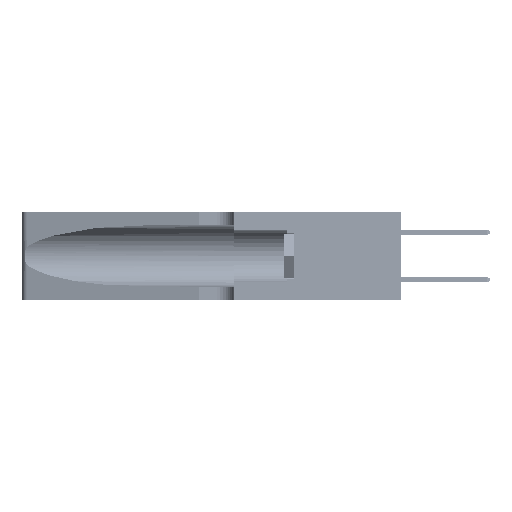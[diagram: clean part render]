
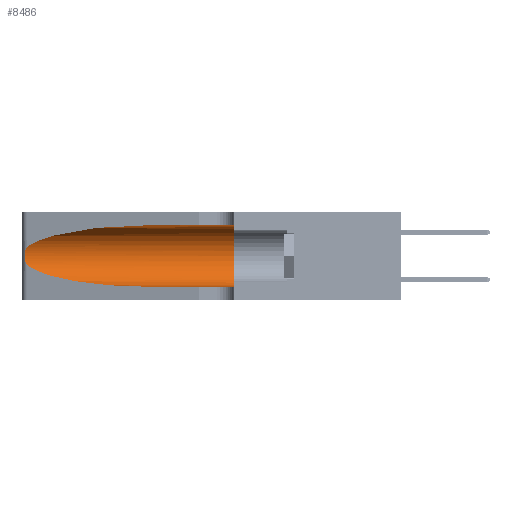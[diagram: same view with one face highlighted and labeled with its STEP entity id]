
A CAD part, left-side view. The second image highlights one B-rep face of the part: STEP entity #8486.
In plain terms, the highlighted cylindrical face has radius 3.308 mm (diameter 6.617 mm), a partial arc.
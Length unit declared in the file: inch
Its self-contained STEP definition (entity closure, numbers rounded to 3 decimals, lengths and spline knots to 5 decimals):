
#449 = CARTESIAN_POINT ( 'NONE',  ( 0.25487, 1.22718, 0.22369 ) ) ;
#981 = VERTEX_POINT ( 'NONE', #46132 ) ;
#1386 = CARTESIAN_POINT ( 'NONE',  ( 0.1305, 0.72297, 0.05475 ) ) ;
#2891 = CARTESIAN_POINT ( 'NONE',  ( 0.26017, 1.23833, 0.17102 ) ) ;
#5799 = CARTESIAN_POINT ( 'NONE',  ( 0.1305, 0.72297, 0.31525 ) ) ;
#6157 = VERTEX_POINT ( 'NONE', #449 ) ;
#6566 = CARTESIAN_POINT ( 'NONE',  ( 0.1305, 1.61858, 0.05475 ) ) ;
#7094 = CARTESIAN_POINT ( 'NONE',  ( 0.25789, 1.23486, 0.15765 ) ) ;
#7376 = CARTESIAN_POINT ( 'NONE',  ( 0.1305, 0.35, 0.185 ) ) ;
#8252 = CARTESIAN_POINT ( 'NONE',  ( 0.1305, 1.61858, 0.31525 ) ) ;
#8486 = ADVANCED_FACE ( 'NONE', ( #23718 ), #43010, .F. ) ;
#9525 = EDGE_CURVE ( 'NONE', #6157, #41247, #24812, .T. ) ;
#10135 = LINE ( 'NONE', #6566, #51354 ) ;
#10443 = ORIENTED_EDGE ( 'NONE', *, *, #43937, .F. ) ;
#10469 = CARTESIAN_POINT ( 'NONE',  ( 0.25487, 1.22718, 0.14631 ) ) ;
#11297 = CARTESIAN_POINT ( 'NONE',  ( 0.25555, 1.22993, 0.14849 ) ) ;
#11585 = DIRECTION ( 'NONE',  ( 0., 0., 1. ) ) ;
#13323 = EDGE_CURVE ( 'NONE', #981, #30240, #10135, .T. ) ;
#14059 = CARTESIAN_POINT ( 'NONE',  ( 0.1305, 0.72297, 0.31525 ) ) ;
#15087 = CARTESIAN_POINT ( 'NONE',  ( 0.25555, 1.22994, 0.2215 ) ) ;
#17076 = EDGE_CURVE ( 'NONE', #32640, #30240, #30531, .T. ) ;
#17966 = CARTESIAN_POINT ( 'NONE',  ( 0.25487, 1.22718, 0.14631 ) ) ;
#19010 = CARTESIAN_POINT ( 'NONE',  ( 0.1305, 1.61858, 0.185 ) ) ;
#19430 = CARTESIAN_POINT ( 'NONE',  ( 0.25787, 1.23484, 0.2124 ) ) ;
#22387 = CARTESIAN_POINT ( 'NONE',  ( 0.25487, 1.22718, 0.22369 ) ) ;
#23558 = CARTESIAN_POINT ( 'NONE',  ( 0.26018, 1.23835, 0.19895 ) ) ;
#23718 = FACE_OUTER_BOUND ( 'NONE', #50709, .T. ) ;
#24812 = B_SPLINE_CURVE_WITH_KNOTS ( 'NONE', 3,
 ( #35809, #15087, #44046, #19430, #48193, #23558, #52320, #27721, #2891, #31877, #7094, #35980, #11297, #40113 ),
 .UNSPECIFIED., .F., .F.,
 ( 4, 2, 2, 2, 2, 2, 4 ),
 ( 0., 0.00027, 0.00053, 0.00107, 0.0016, 0.00187, 0.00214 ),
 .UNSPECIFIED. ) ;
#25720 = ORIENTED_EDGE ( 'NONE', *, *, #41155, .T. ) ;
#26239 = CARTESIAN_POINT ( 'NONE',  ( 0.18966, 0.96281, 0.05475 ) ) ;
#27721 = CARTESIAN_POINT ( 'NONE',  ( 0.26075, 1.23896, 0.178 ) ) ;
#29228 = ORIENTED_EDGE ( 'NONE', *, *, #9525, .T. ) ;
#29421 =( BOUNDED_CURVE ( )  B_SPLINE_CURVE ( 3, ( #17966, #46732, #26239, #1386 ),
 .UNSPECIFIED., .F., .T. ) 
 B_SPLINE_CURVE_WITH_KNOTS ( ( 4, 4 ),
 ( 3.44316, 4.71239 ),
 .UNSPECIFIED. ) 
 CURVE ( )  GEOMETRIC_REPRESENTATION_ITEM ( )  RATIONAL_B_SPLINE_CURVE ( ( 1., 0.87, 0.87, 1. ) ) 
 REPRESENTATION_ITEM ( '' )  );
#30240 = VERTEX_POINT ( 'NONE', #32437 ) ;
#30531 = CIRCLE ( 'NONE', #51587, 0.13025 ) ;
#31877 = CARTESIAN_POINT ( 'NONE',  ( 0.25856, 1.23593, 0.16098 ) ) ;
#32437 = CARTESIAN_POINT ( 'NONE',  ( 0.1305, 0.35, 0.05475 ) ) ;
#32640 = VERTEX_POINT ( 'NONE', #41630 ) ;
#34640 = CARTESIAN_POINT ( 'NONE',  ( 0.18966, 0.96281, 0.31525 ) ) ;
#35809 = CARTESIAN_POINT ( 'NONE',  ( 0.25487, 1.22718, 0.22369 ) ) ;
#35980 = CARTESIAN_POINT ( 'NONE',  ( 0.25639, 1.23186, 0.15144 ) ) ;
#36270 = DIRECTION ( 'NONE',  ( 0., 1., 0. ) ) ;
#38924 =( BOUNDED_CURVE ( )  B_SPLINE_CURVE ( 3, ( #14059, #34640, #47025, #22387 ),
 .UNSPECIFIED., .F., .F. ) 
 B_SPLINE_CURVE_WITH_KNOTS ( ( 4, 4 ),
 ( 1.5708, 2.84003 ),
 .UNSPECIFIED. ) 
 CURVE ( )  GEOMETRIC_REPRESENTATION_ITEM ( )  RATIONAL_B_SPLINE_CURVE ( ( 1., 0.87, 0.87, 1. ) ) 
 REPRESENTATION_ITEM ( '' )  );
#39523 = LINE ( 'NONE', #8252, #49156 ) ;
#39600 = DIRECTION ( 'NONE',  ( 0., -1., 0. ) ) ;
#40113 = CARTESIAN_POINT ( 'NONE',  ( 0.25487, 1.22718, 0.14631 ) ) ;
#40343 = ORIENTED_EDGE ( 'NONE', *, *, #17076, .F. ) ;
#40459 = EDGE_CURVE ( 'NONE', #41247, #981, #29421, .T. ) ;
#41155 = EDGE_CURVE ( 'NONE', #50960, #6157, #38924, .T. ) ;
#41226 = DIRECTION ( 'NONE',  ( 0., -1., 0. ) ) ;
#41247 = VERTEX_POINT ( 'NONE', #10469 ) ;
#41630 = CARTESIAN_POINT ( 'NONE',  ( 0.1305, 0.35, 0.31525 ) ) ;
#43010 = CYLINDRICAL_SURFACE ( 'NONE', #45846, 0.13025 ) ;
#43631 = DIRECTION ( 'NONE',  ( 0., -1., 0. ) ) ;
#43907 = ORIENTED_EDGE ( 'NONE', *, *, #13323, .T. ) ;
#43937 = EDGE_CURVE ( 'NONE', #50960, #32640, #39523, .T. ) ;
#44046 = CARTESIAN_POINT ( 'NONE',  ( 0.25639, 1.23184, 0.21858 ) ) ;
#45846 = AXIS2_PLACEMENT_3D ( 'NONE', #19010, #43631, #51559 ) ;
#46034 = ORIENTED_EDGE ( 'NONE', *, *, #40459, .T. ) ;
#46132 = CARTESIAN_POINT ( 'NONE',  ( 0.1305, 0.72297, 0.05475 ) ) ;
#46732 = CARTESIAN_POINT ( 'NONE',  ( 0.2373, 1.15595, 0.08982 ) ) ;
#47025 = CARTESIAN_POINT ( 'NONE',  ( 0.2373, 1.15595, 0.28018 ) ) ;
#48193 = CARTESIAN_POINT ( 'NONE',  ( 0.25854, 1.2359, 0.20912 ) ) ;
#49156 = VECTOR ( 'NONE', #41226, 39.37008 ) ;
#50709 = EDGE_LOOP ( 'NONE', ( #25720, #29228, #46034, #43907, #40343, #10443 ) ) ;
#50960 = VERTEX_POINT ( 'NONE', #5799 ) ;
#51354 = VECTOR ( 'NONE', #39600, 39.37008 ) ;
#51559 = DIRECTION ( 'NONE',  ( 0., 0., -1. ) ) ;
#51587 = AXIS2_PLACEMENT_3D ( 'NONE', #7376, #36270, #11585 ) ;
#52320 = CARTESIAN_POINT ( 'NONE',  ( 0.26075, 1.23896, 0.19203 ) ) ;
